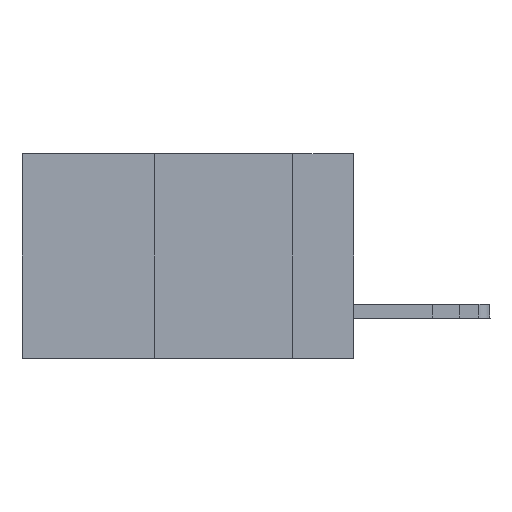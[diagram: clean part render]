
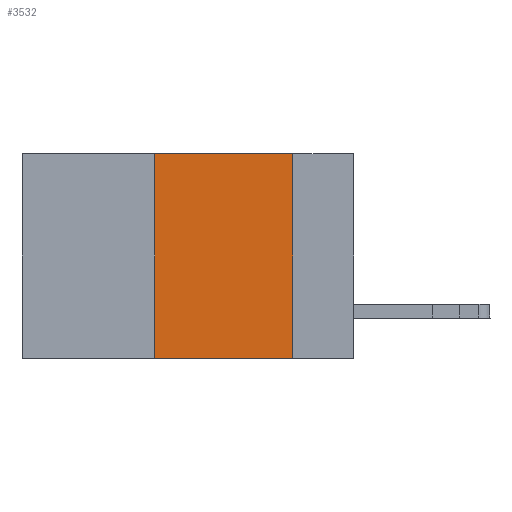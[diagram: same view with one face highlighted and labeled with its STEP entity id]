
A CAD part, left-side view. The second image highlights one B-rep face of the part: STEP entity #3532.
In plain terms, the highlighted planar face has unit normal (-1, 0, 0).
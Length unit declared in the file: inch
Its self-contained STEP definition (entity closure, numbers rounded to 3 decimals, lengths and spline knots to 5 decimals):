
#95 = LINE ( 'NONE', #5642, #12695 ) ;
#889 = PLANE ( 'NONE',  #2822 ) ;
#1315 = VECTOR ( 'NONE', #3024, 39.37008 ) ;
#1343 = EDGE_LOOP ( 'NONE', ( #22663, #6873, #23033, #3586 ) ) ;
#1728 = DIRECTION ( 'NONE',  ( 0., -1., 0. ) ) ;
#2007 = DIRECTION ( 'NONE',  ( 0., -1., 0. ) ) ;
#2161 = CARTESIAN_POINT ( 'NONE',  ( 0., 0.36, 0. ) ) ;
#2822 = AXIS2_PLACEMENT_3D ( 'NONE', #8606, #15933, #16025 ) ;
#3024 = DIRECTION ( 'NONE',  ( 0., 0., 1. ) ) ;
#3532 = ADVANCED_FACE ( 'NONE', ( #9208 ), #889, .F. ) ;
#3586 = ORIENTED_EDGE ( 'NONE', *, *, #3838, .T. ) ;
#3838 = EDGE_CURVE ( 'NONE', #5111, #16850, #95, .T. ) ;
#3883 = CARTESIAN_POINT ( 'NONE',  ( 0., 0.11, -0.37 ) ) ;
#4404 = LINE ( 'NONE', #22378, #17610 ) ;
#5111 = VERTEX_POINT ( 'NONE', #15769 ) ;
#5367 = LINE ( 'NONE', #9842, #22911 ) ;
#5642 = CARTESIAN_POINT ( 'NONE',  ( 0., 0.6, -0.37 ) ) ;
#6175 = EDGE_CURVE ( 'NONE', #13885, #18301, #4404, .T. ) ;
#6873 = ORIENTED_EDGE ( 'NONE', *, *, #6175, .F. ) ;
#8606 = CARTESIAN_POINT ( 'NONE',  ( 0., 0.6, 0. ) ) ;
#8646 = LINE ( 'NONE', #2161, #1315 ) ;
#9208 = FACE_OUTER_BOUND ( 'NONE', #1343, .T. ) ;
#9842 = CARTESIAN_POINT ( 'NONE',  ( 0., 0.11, 0. ) ) ;
#12695 = VECTOR ( 'NONE', #2007, 39.37008 ) ;
#13146 = EDGE_CURVE ( 'NONE', #18301, #16850, #5367, .T. ) ;
#13513 = DIRECTION ( 'NONE',  ( 0., 0., -1. ) ) ;
#13885 = VERTEX_POINT ( 'NONE', #17621 ) ;
#14841 = EDGE_CURVE ( 'NONE', #5111, #13885, #8646, .T. ) ;
#14988 = CARTESIAN_POINT ( 'NONE',  ( 0., 0.11, 0. ) ) ;
#15769 = CARTESIAN_POINT ( 'NONE',  ( 0., 0.36, -0.37 ) ) ;
#15933 = DIRECTION ( 'NONE',  ( 1., 0., 0. ) ) ;
#16025 = DIRECTION ( 'NONE',  ( 0., 0., -1. ) ) ;
#16850 = VERTEX_POINT ( 'NONE', #3883 ) ;
#17610 = VECTOR ( 'NONE', #1728, 39.37008 ) ;
#17621 = CARTESIAN_POINT ( 'NONE',  ( 0., 0.36, 0. ) ) ;
#18301 = VERTEX_POINT ( 'NONE', #14988 ) ;
#22378 = CARTESIAN_POINT ( 'NONE',  ( 0., 0.6, 0. ) ) ;
#22663 = ORIENTED_EDGE ( 'NONE', *, *, #13146, .F. ) ;
#22911 = VECTOR ( 'NONE', #13513, 39.37008 ) ;
#23033 = ORIENTED_EDGE ( 'NONE', *, *, #14841, .F. ) ;
